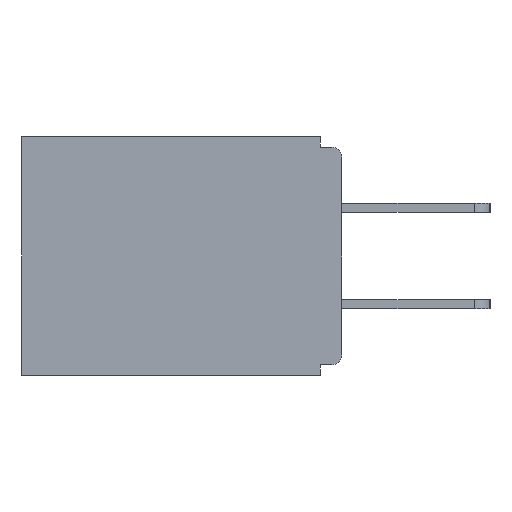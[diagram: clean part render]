
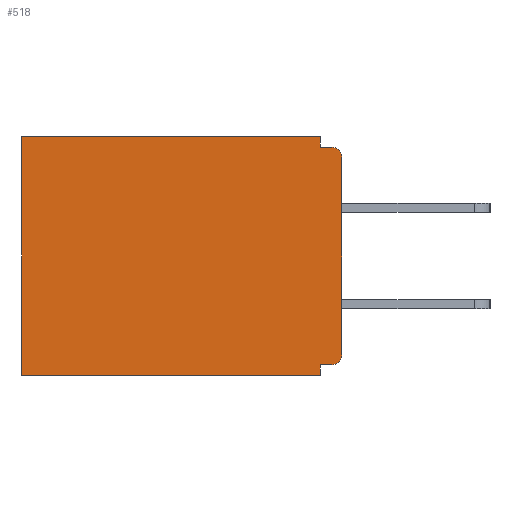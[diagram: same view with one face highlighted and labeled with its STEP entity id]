
A CAD part, left-side view. The second image highlights one B-rep face of the part: STEP entity #518.
In plain terms, the highlighted planar face has unit normal (-1, 0, 0).
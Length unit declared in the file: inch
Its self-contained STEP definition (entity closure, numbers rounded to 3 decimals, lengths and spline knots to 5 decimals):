
#52 = VECTOR ( 'NONE', #6981, 39.37008 ) ;
#104 = DIRECTION ( 'NONE',  ( 0., 0., -1. ) ) ;
#398 = CARTESIAN_POINT ( 'NONE',  ( 0.298, 0., -0.03 ) ) ;
#518 = ADVANCED_FACE ( 'NONE', ( #12830 ), #11146, .F. ) ;
#550 = VECTOR ( 'NONE', #7083, 39.37008 ) ;
#640 = ORIENTED_EDGE ( 'NONE', *, *, #12588, .T. ) ;
#660 = ORIENTED_EDGE ( 'NONE', *, *, #1701, .T. ) ;
#680 = CARTESIAN_POINT ( 'NONE',  ( 0.298, 0.031, 0. ) ) ;
#917 = DIRECTION ( 'NONE',  ( 0., 0., -1. ) ) ;
#947 = DIRECTION ( 'NONE',  ( 0., 1., 0. ) ) ;
#1151 = EDGE_LOOP ( 'NONE', ( #3875, #6096, #5884, #2622, #660, #9315, #8125, #4077, #640, #12863 ) ) ;
#1460 = VECTOR ( 'NONE', #5550, 39.37008 ) ;
#1701 = EDGE_CURVE ( 'NONE', #3964, #7918, #5057, .T. ) ;
#1757 = EDGE_CURVE ( 'NONE', #2545, #3964, #8273, .T. ) ;
#1784 = LINE ( 'NONE', #12772, #1460 ) ;
#2019 = CARTESIAN_POINT ( 'NONE',  ( 0.298, 0.015, -0.03 ) ) ;
#2545 = VERTEX_POINT ( 'NONE', #680 ) ;
#2622 = ORIENTED_EDGE ( 'NONE', *, *, #1757, .T. ) ;
#2646 = AXIS2_PLACEMENT_3D ( 'NONE', #10792, #6783, #12935 ) ;
#3234 = LINE ( 'NONE', #4485, #12747 ) ;
#3689 = CARTESIAN_POINT ( 'NONE',  ( 0.298, 0.46, -0.343 ) ) ;
#3875 = ORIENTED_EDGE ( 'NONE', *, *, #10097, .T. ) ;
#3932 = VECTOR ( 'NONE', #4040, 39.37008 ) ;
#3964 = VERTEX_POINT ( 'NONE', #12255 ) ;
#4040 = DIRECTION ( 'NONE',  ( 0., 1., 0. ) ) ;
#4077 = ORIENTED_EDGE ( 'NONE', *, *, #4344, .F. ) ;
#4344 = EDGE_CURVE ( 'NONE', #5920, #6208, #1784, .T. ) ;
#4485 = CARTESIAN_POINT ( 'NONE',  ( 0.298, 0., -0.015 ) ) ;
#4773 = AXIS2_PLACEMENT_3D ( 'NONE', #13114, #6900, #10068 ) ;
#5057 = LINE ( 'NONE', #5067, #52 ) ;
#5067 = CARTESIAN_POINT ( 'NONE',  ( 0.298, 0.46, 0. ) ) ;
#5245 = VECTOR ( 'NONE', #947, 39.37008 ) ;
#5321 = DIRECTION ( 'NONE',  ( 0., -1., 0. ) ) ;
#5550 = DIRECTION ( 'NONE',  ( 0., 1., 0. ) ) ;
#5748 = VERTEX_POINT ( 'NONE', #11317 ) ;
#5884 = ORIENTED_EDGE ( 'NONE', *, *, #12891, .F. ) ;
#5920 = VERTEX_POINT ( 'NONE', #6837 ) ;
#5950 = CARTESIAN_POINT ( 'NONE',  ( 0.298, 0.031, -0.015 ) ) ;
#6096 = ORIENTED_EDGE ( 'NONE', *, *, #10145, .F. ) ;
#6208 = VERTEX_POINT ( 'NONE', #8426 ) ;
#6331 = VERTEX_POINT ( 'NONE', #5950 ) ;
#6363 = VECTOR ( 'NONE', #917, 39.37008 ) ;
#6521 = CARTESIAN_POINT ( 'NONE',  ( 0.298, 0.015, -0.015 ) ) ;
#6783 = DIRECTION ( 'NONE',  ( -1., 0., 0. ) ) ;
#6837 = CARTESIAN_POINT ( 'NONE',  ( 0.298, 0.015, -0.328 ) ) ;
#6900 = DIRECTION ( 'NONE',  ( 1., 0., 0. ) ) ;
#6981 = DIRECTION ( 'NONE',  ( 0., 0., -1. ) ) ;
#7083 = DIRECTION ( 'NONE',  ( 0., 0., -1. ) ) ;
#7142 = CIRCLE ( 'NONE', #2646, 0.015 ) ;
#7795 = CARTESIAN_POINT ( 'NONE',  ( 0.298, 0.031, -0.343 ) ) ;
#7918 = VERTEX_POINT ( 'NONE', #3689 ) ;
#7965 = LINE ( 'NONE', #11036, #6363 ) ;
#8125 = ORIENTED_EDGE ( 'NONE', *, *, #8329, .F. ) ;
#8182 = CARTESIAN_POINT ( 'NONE',  ( 0.298, 0., -0.343 ) ) ;
#8221 = AXIS2_PLACEMENT_3D ( 'NONE', #2019, #9310, #104 ) ;
#8273 = LINE ( 'NONE', #11220, #3932 ) ;
#8317 = VERTEX_POINT ( 'NONE', #12493 ) ;
#8329 = EDGE_CURVE ( 'NONE', #6208, #8317, #8907, .T. ) ;
#8426 = CARTESIAN_POINT ( 'NONE',  ( 0.298, 0.031, -0.328 ) ) ;
#8907 = LINE ( 'NONE', #9474, #550 ) ;
#9250 = VERTEX_POINT ( 'NONE', #398 ) ;
#9310 = DIRECTION ( 'NONE',  ( -1., 0., 0. ) ) ;
#9315 = ORIENTED_EDGE ( 'NONE', *, *, #12284, .F. ) ;
#9474 = CARTESIAN_POINT ( 'NONE',  ( 0.298, 0.031, -0.343 ) ) ;
#10068 = DIRECTION ( 'NONE',  ( 0., 0., -1. ) ) ;
#10097 = EDGE_CURVE ( 'NONE', #9250, #10376, #12411, .T. ) ;
#10145 = EDGE_CURVE ( 'NONE', #6331, #10376, #3234, .T. ) ;
#10376 = VERTEX_POINT ( 'NONE', #6521 ) ;
#10535 = VECTOR ( 'NONE', #13001, 39.37008 ) ;
#10792 = CARTESIAN_POINT ( 'NONE',  ( 0.298, 0.015, -0.313 ) ) ;
#10867 = LINE ( 'NONE', #7795, #10535 ) ;
#11036 = CARTESIAN_POINT ( 'NONE',  ( 0.298, 0., 0. ) ) ;
#11146 = PLANE ( 'NONE',  #4773 ) ;
#11220 = CARTESIAN_POINT ( 'NONE',  ( 0.298, 0., 0. ) ) ;
#11317 = CARTESIAN_POINT ( 'NONE',  ( 0.298, 0., -0.313 ) ) ;
#12255 = CARTESIAN_POINT ( 'NONE',  ( 0.298, 0.46, 0. ) ) ;
#12284 = EDGE_CURVE ( 'NONE', #8317, #7918, #13175, .T. ) ;
#12411 = CIRCLE ( 'NONE', #8221, 0.015 ) ;
#12493 = CARTESIAN_POINT ( 'NONE',  ( 0.298, 0.031, -0.343 ) ) ;
#12588 = EDGE_CURVE ( 'NONE', #5920, #5748, #7142, .T. ) ;
#12747 = VECTOR ( 'NONE', #5321, 39.37008 ) ;
#12772 = CARTESIAN_POINT ( 'NONE',  ( 0.298, 0., -0.328 ) ) ;
#12830 = FACE_OUTER_BOUND ( 'NONE', #1151, .T. ) ;
#12863 = ORIENTED_EDGE ( 'NONE', *, *, #13125, .F. ) ;
#12891 = EDGE_CURVE ( 'NONE', #2545, #6331, #10867, .T. ) ;
#12935 = DIRECTION ( 'NONE',  ( 0., 0., -1. ) ) ;
#13001 = DIRECTION ( 'NONE',  ( 0., 0., -1. ) ) ;
#13114 = CARTESIAN_POINT ( 'NONE',  ( 0.298, 0., 0. ) ) ;
#13125 = EDGE_CURVE ( 'NONE', #9250, #5748, #7965, .T. ) ;
#13175 = LINE ( 'NONE', #8182, #5245 ) ;
